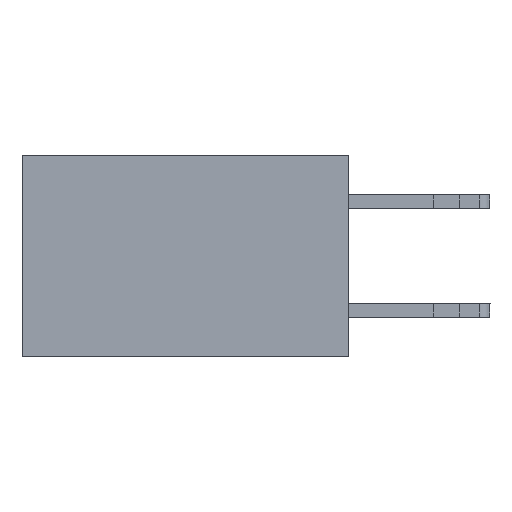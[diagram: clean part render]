
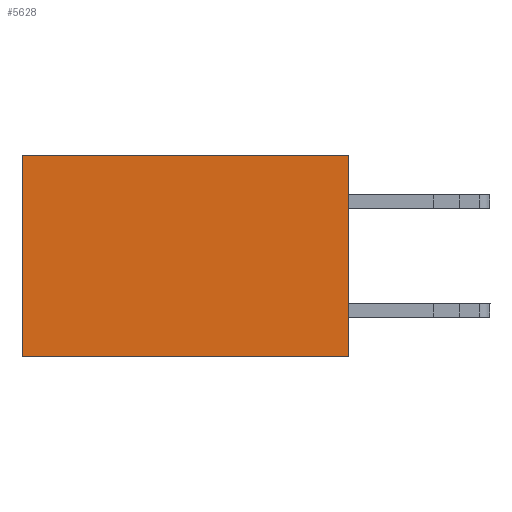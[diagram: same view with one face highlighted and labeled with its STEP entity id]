
A CAD part, left-side view. The second image highlights one B-rep face of the part: STEP entity #5628.
In plain terms, the highlighted planar face has unit normal (-1, 0, 0).
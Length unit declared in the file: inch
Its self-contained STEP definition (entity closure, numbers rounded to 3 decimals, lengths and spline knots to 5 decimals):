
#1162 = LINE ( 'NONE', #15073, #23440 ) ;
#1402 = ORIENTED_EDGE ( 'NONE', *, *, #1494, .T. ) ;
#1494 = EDGE_CURVE ( 'NONE', #5620, #12332, #17616, .T. ) ;
#1768 = AXIS2_PLACEMENT_3D ( 'NONE', #12731, #14651, #16933 ) ;
#2122 = EDGE_CURVE ( 'NONE', #13727, #5620, #6660, .T. ) ;
#3326 = CARTESIAN_POINT ( 'NONE',  ( 0.298, 0., 0. ) ) ;
#3687 = LINE ( 'NONE', #3326, #15990 ) ;
#4982 = DIRECTION ( 'NONE',  ( 0., 1., 0. ) ) ;
#5620 = VERTEX_POINT ( 'NONE', #19052 ) ;
#5628 = ADVANCED_FACE ( 'NONE', ( #17407 ), #27792, .F. ) ;
#6660 = LINE ( 'NONE', #9550, #26881 ) ;
#7695 = CARTESIAN_POINT ( 'NONE',  ( 0.298, 0.6, -0.37 ) ) ;
#9550 = CARTESIAN_POINT ( 'NONE',  ( 0.298, 0., 0. ) ) ;
#11398 = VERTEX_POINT ( 'NONE', #14732 ) ;
#12332 = VERTEX_POINT ( 'NONE', #7695 ) ;
#12731 = CARTESIAN_POINT ( 'NONE',  ( 0.298, 0., 0. ) ) ;
#13727 = VERTEX_POINT ( 'NONE', #23473 ) ;
#14651 = DIRECTION ( 'NONE',  ( 1., 0., 0. ) ) ;
#14732 = CARTESIAN_POINT ( 'NONE',  ( 0.298, 0., -0.37 ) ) ;
#15073 = CARTESIAN_POINT ( 'NONE',  ( 0.298, 0., -0.37 ) ) ;
#15548 = VECTOR ( 'NONE', #15751, 39.37008 ) ;
#15751 = DIRECTION ( 'NONE',  ( 0., 0., -1. ) ) ;
#15990 = VECTOR ( 'NONE', #27189, 39.37008 ) ;
#16656 = EDGE_LOOP ( 'NONE', ( #1402, #17077, #25079, #22728 ) ) ;
#16933 = DIRECTION ( 'NONE',  ( 0., 0., -1. ) ) ;
#17077 = ORIENTED_EDGE ( 'NONE', *, *, #27563, .F. ) ;
#17407 = FACE_OUTER_BOUND ( 'NONE', #16656, .T. ) ;
#17616 = LINE ( 'NONE', #20007, #15548 ) ;
#19052 = CARTESIAN_POINT ( 'NONE',  ( 0.298, 0.6, 0. ) ) ;
#20007 = CARTESIAN_POINT ( 'NONE',  ( 0.298, 0.6, 0. ) ) ;
#21679 = DIRECTION ( 'NONE',  ( 0., 1., 0. ) ) ;
#22728 = ORIENTED_EDGE ( 'NONE', *, *, #2122, .T. ) ;
#23440 = VECTOR ( 'NONE', #21679, 39.37008 ) ;
#23473 = CARTESIAN_POINT ( 'NONE',  ( 0.298, 0., 0. ) ) ;
#24904 = EDGE_CURVE ( 'NONE', #13727, #11398, #3687, .T. ) ;
#25079 = ORIENTED_EDGE ( 'NONE', *, *, #24904, .F. ) ;
#26881 = VECTOR ( 'NONE', #4982, 39.37008 ) ;
#27189 = DIRECTION ( 'NONE',  ( 0., 0., -1. ) ) ;
#27563 = EDGE_CURVE ( 'NONE', #11398, #12332, #1162, .T. ) ;
#27792 = PLANE ( 'NONE',  #1768 ) ;
